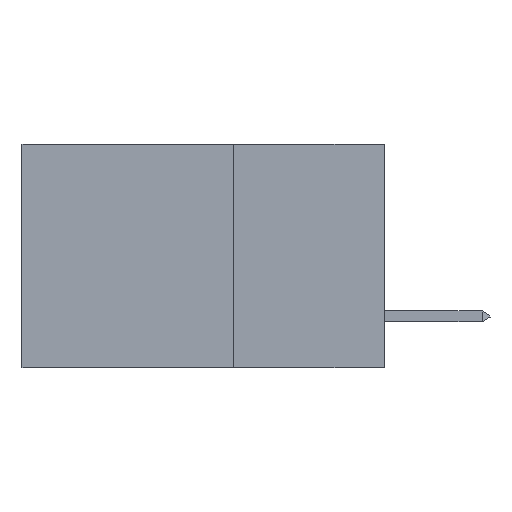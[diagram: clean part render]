
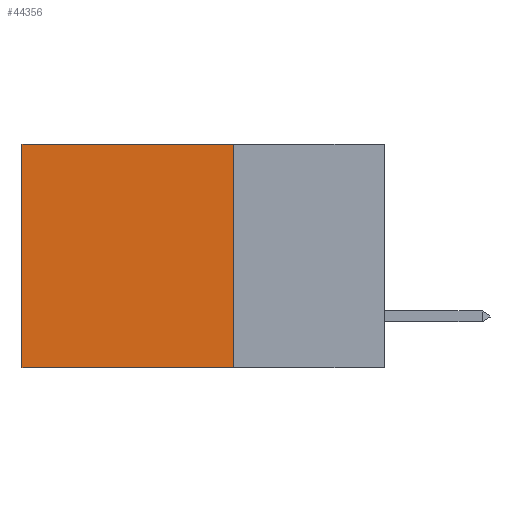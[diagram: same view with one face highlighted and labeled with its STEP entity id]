
A CAD part, left-side view. The second image highlights one B-rep face of the part: STEP entity #44356.
In plain terms, the highlighted planar face has unit normal (-1, 0, 0).
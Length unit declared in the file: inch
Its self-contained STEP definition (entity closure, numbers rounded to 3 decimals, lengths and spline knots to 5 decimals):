
#44 = EDGE_CURVE ( 'NONE', #1307, #28362, #11800, .T. ) ;
#440 = ORIENTED_EDGE ( 'NONE', *, *, #36339, .T. ) ;
#1307 = VERTEX_POINT ( 'NONE', #13960 ) ;
#1443 = CARTESIAN_POINT ( 'NONE',  ( 0.2875, 0.25, 0. ) ) ;
#4527 = CARTESIAN_POINT ( 'NONE',  ( 0.2875, 0.6, 0. ) ) ;
#4660 = FACE_OUTER_BOUND ( 'NONE', #45723, .T. ) ;
#7062 = DIRECTION ( 'NONE',  ( 0., 1., 0. ) ) ;
#9941 = CARTESIAN_POINT ( 'NONE',  ( 0.2875, 0.25, 0. ) ) ;
#11800 = LINE ( 'NONE', #9941, #39540 ) ;
#13960 = CARTESIAN_POINT ( 'NONE',  ( 0.2875, 0.25, 0. ) ) ;
#16539 = LINE ( 'NONE', #32875, #24299 ) ;
#16696 = DIRECTION ( 'NONE',  ( 0., 0., -1. ) ) ;
#17182 = CARTESIAN_POINT ( 'NONE',  ( 0.2875, 0.25, 0. ) ) ;
#18710 = LINE ( 'NONE', #25974, #47119 ) ;
#23634 = EDGE_CURVE ( 'NONE', #28362, #34061, #18710, .T. ) ;
#24299 = VECTOR ( 'NONE', #44275, 39.37008 ) ;
#25974 = CARTESIAN_POINT ( 'NONE',  ( 0.2875, 0.25, -0.37 ) ) ;
#27347 = AXIS2_PLACEMENT_3D ( 'NONE', #1443, #39309, #16696 ) ;
#28362 = VERTEX_POINT ( 'NONE', #31010 ) ;
#28811 = DIRECTION ( 'NONE',  ( 0., 0., -1. ) ) ;
#30125 = ORIENTED_EDGE ( 'NONE', *, *, #23634, .F. ) ;
#31010 = CARTESIAN_POINT ( 'NONE',  ( 0.2875, 0.25, -0.37 ) ) ;
#32875 = CARTESIAN_POINT ( 'NONE',  ( 0.2875, 0.6, 0. ) ) ;
#34061 = VERTEX_POINT ( 'NONE', #39747 ) ;
#35509 = PLANE ( 'NONE',  #27347 ) ;
#36339 = EDGE_CURVE ( 'NONE', #1307, #41467, #47761, .T. ) ;
#37681 = VECTOR ( 'NONE', #47397, 39.37008 ) ;
#39309 = DIRECTION ( 'NONE',  ( 1., 0., 0. ) ) ;
#39540 = VECTOR ( 'NONE', #28811, 39.37008 ) ;
#39747 = CARTESIAN_POINT ( 'NONE',  ( 0.2875, 0.6, -0.37 ) ) ;
#41467 = VERTEX_POINT ( 'NONE', #4527 ) ;
#44275 = DIRECTION ( 'NONE',  ( 0., 0., -1. ) ) ;
#44356 = ADVANCED_FACE ( 'NONE', ( #4660 ), #35509, .F. ) ;
#45723 = EDGE_LOOP ( 'NONE', ( #46198, #30125, #47327, #440 ) ) ;
#46198 = ORIENTED_EDGE ( 'NONE', *, *, #46395, .T. ) ;
#46395 = EDGE_CURVE ( 'NONE', #41467, #34061, #16539, .T. ) ;
#47119 = VECTOR ( 'NONE', #7062, 39.37008 ) ;
#47327 = ORIENTED_EDGE ( 'NONE', *, *, #44, .F. ) ;
#47397 = DIRECTION ( 'NONE',  ( 0., 1., 0. ) ) ;
#47761 = LINE ( 'NONE', #17182, #37681 ) ;
